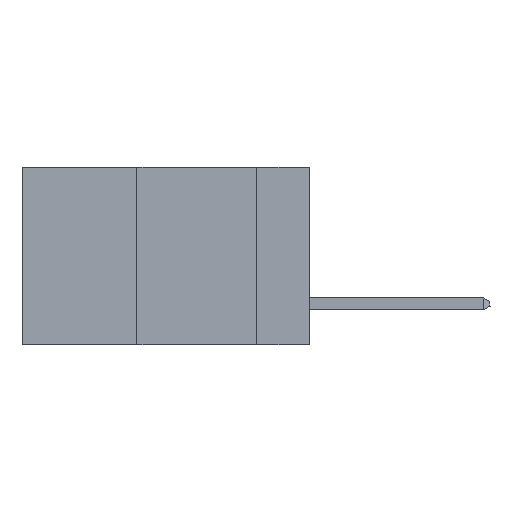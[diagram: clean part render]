
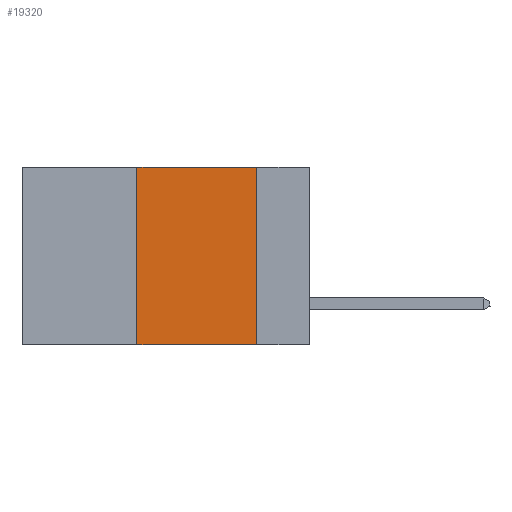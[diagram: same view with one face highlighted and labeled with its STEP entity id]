
A CAD part, left-side view. The second image highlights one B-rep face of the part: STEP entity #19320.
In plain terms, the highlighted planar face has unit normal (-1, 0, 0).
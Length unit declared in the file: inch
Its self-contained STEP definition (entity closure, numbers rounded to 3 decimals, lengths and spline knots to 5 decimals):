
#144 = EDGE_CURVE ( 'NONE', #25260, #4963, #26484, .T. ) ;
#543 = CARTESIAN_POINT ( 'NONE',  ( 0., 0.11, -0.37 ) ) ;
#1886 = VERTEX_POINT ( 'NONE', #3712 ) ;
#2211 = EDGE_LOOP ( 'NONE', ( #20959, #36915, #23644, #10573 ) ) ;
#2292 = AXIS2_PLACEMENT_3D ( 'NONE', #31263, #15846, #18547 ) ;
#3712 = CARTESIAN_POINT ( 'NONE',  ( 0., 0.11, 0. ) ) ;
#4051 = LINE ( 'NONE', #37351, #24392 ) ;
#4921 = CARTESIAN_POINT ( 'NONE',  ( 0., 0.6, -0.37 ) ) ;
#4963 = VERTEX_POINT ( 'NONE', #543 ) ;
#5640 = DIRECTION ( 'NONE',  ( 0., -1., 0. ) ) ;
#5789 = FACE_OUTER_BOUND ( 'NONE', #2211, .T. ) ;
#6385 = CARTESIAN_POINT ( 'NONE',  ( 0., 0.36, 0. ) ) ;
#6720 = LINE ( 'NONE', #15744, #15471 ) ;
#6799 = EDGE_CURVE ( 'NONE', #28903, #1886, #4051, .T. ) ;
#10573 = ORIENTED_EDGE ( 'NONE', *, *, #144, .T. ) ;
#11647 = EDGE_CURVE ( 'NONE', #25260, #28903, #16742, .T. ) ;
#11914 = VECTOR ( 'NONE', #21507, 39.37008 ) ;
#15471 = VECTOR ( 'NONE', #24668, 39.37008 ) ;
#15744 = CARTESIAN_POINT ( 'NONE',  ( 0., 0.11, 0. ) ) ;
#15846 = DIRECTION ( 'NONE',  ( 1., 0., 0. ) ) ;
#16706 = CARTESIAN_POINT ( 'NONE',  ( 0., 0.36, -0.37 ) ) ;
#16742 = LINE ( 'NONE', #6385, #11914 ) ;
#17374 = VECTOR ( 'NONE', #26040, 39.37008 ) ;
#17894 = EDGE_CURVE ( 'NONE', #1886, #4963, #6720, .T. ) ;
#18547 = DIRECTION ( 'NONE',  ( 0., 0., -1. ) ) ;
#18661 = PLANE ( 'NONE',  #2292 ) ;
#19320 = ADVANCED_FACE ( 'NONE', ( #5789 ), #18661, .F. ) ;
#20959 = ORIENTED_EDGE ( 'NONE', *, *, #17894, .F. ) ;
#21507 = DIRECTION ( 'NONE',  ( 0., 0., 1. ) ) ;
#23644 = ORIENTED_EDGE ( 'NONE', *, *, #11647, .F. ) ;
#24392 = VECTOR ( 'NONE', #5640, 39.37008 ) ;
#24668 = DIRECTION ( 'NONE',  ( 0., 0., -1. ) ) ;
#25260 = VERTEX_POINT ( 'NONE', #16706 ) ;
#26040 = DIRECTION ( 'NONE',  ( 0., -1., 0. ) ) ;
#26484 = LINE ( 'NONE', #4921, #17374 ) ;
#28903 = VERTEX_POINT ( 'NONE', #34870 ) ;
#31263 = CARTESIAN_POINT ( 'NONE',  ( 0., 0.6, 0. ) ) ;
#34870 = CARTESIAN_POINT ( 'NONE',  ( 0., 0.36, 0. ) ) ;
#36915 = ORIENTED_EDGE ( 'NONE', *, *, #6799, .F. ) ;
#37351 = CARTESIAN_POINT ( 'NONE',  ( 0., 0.6, 0. ) ) ;
